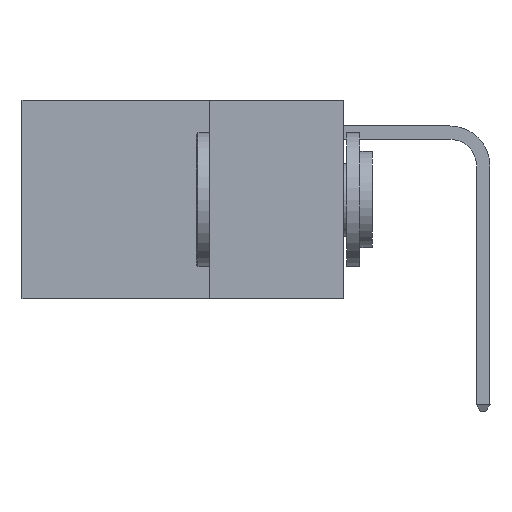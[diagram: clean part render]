
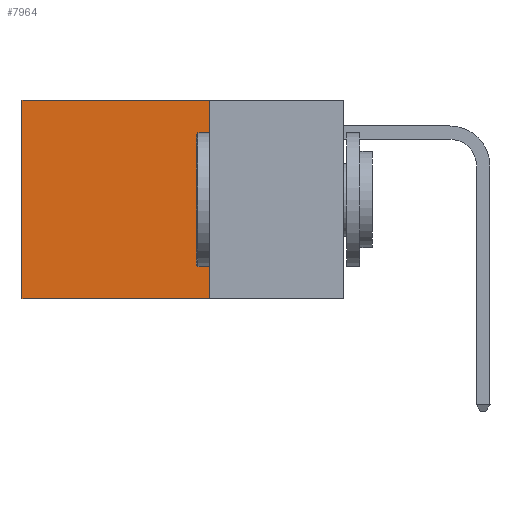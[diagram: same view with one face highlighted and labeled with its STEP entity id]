
A CAD part, left-side view. The second image highlights one B-rep face of the part: STEP entity #7964.
In plain terms, the highlighted planar face has unit normal (-1, 0, 0).
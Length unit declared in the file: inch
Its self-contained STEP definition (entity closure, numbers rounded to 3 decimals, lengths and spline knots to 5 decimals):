
#1226 = CARTESIAN_POINT ( 'NONE',  ( 0.2625, 0.25, 0. ) ) ;
#1303 = FACE_OUTER_BOUND ( 'NONE', #14444, .T. ) ;
#2228 = LINE ( 'NONE', #5620, #14779 ) ;
#3333 = DIRECTION ( 'NONE',  ( 0., 0., -1. ) ) ;
#3368 = EDGE_CURVE ( 'NONE', #9270, #14042, #2228, .T. ) ;
#3761 = EDGE_CURVE ( 'NONE', #9270, #8616, #7648, .T. ) ;
#3836 = DIRECTION ( 'NONE',  ( 0., 1., 0. ) ) ;
#4022 = CARTESIAN_POINT ( 'NONE',  ( 0.2625, 0.6, -0.37 ) ) ;
#4247 = VECTOR ( 'NONE', #3836, 39.37008 ) ;
#4575 = CARTESIAN_POINT ( 'NONE',  ( 0.2625, 0.6, 0. ) ) ;
#4822 = DIRECTION ( 'NONE',  ( 0., 0., -1. ) ) ;
#4838 = PLANE ( 'NONE',  #9672 ) ;
#5023 = CARTESIAN_POINT ( 'NONE',  ( 0.2625, 0.25, -0.37 ) ) ;
#5375 = VECTOR ( 'NONE', #4822, 39.37008 ) ;
#5493 = ORIENTED_EDGE ( 'NONE', *, *, #15145, .F. ) ;
#5620 = CARTESIAN_POINT ( 'NONE',  ( 0.2625, 0.25, 0. ) ) ;
#6087 = CARTESIAN_POINT ( 'NONE',  ( 0.2625, 0.6, 0. ) ) ;
#6207 = CARTESIAN_POINT ( 'NONE',  ( 0.2625, 0.25, 0. ) ) ;
#6238 = LINE ( 'NONE', #6087, #5375 ) ;
#7437 = DIRECTION ( 'NONE',  ( 1., 0., 0. ) ) ;
#7648 = LINE ( 'NONE', #10483, #7732 ) ;
#7732 = VECTOR ( 'NONE', #11745, 39.37008 ) ;
#7964 = ADVANCED_FACE ( 'NONE', ( #1303 ), #4838, .F. ) ;
#8307 = EDGE_CURVE ( 'NONE', #8616, #10285, #6238, .T. ) ;
#8616 = VERTEX_POINT ( 'NONE', #4575 ) ;
#9270 = VERTEX_POINT ( 'NONE', #6207 ) ;
#9672 = AXIS2_PLACEMENT_3D ( 'NONE', #1226, #7437, #11139 ) ;
#10285 = VERTEX_POINT ( 'NONE', #4022 ) ;
#10483 = CARTESIAN_POINT ( 'NONE',  ( 0.2625, 0.25, 0. ) ) ;
#11139 = DIRECTION ( 'NONE',  ( 0., 0., -1. ) ) ;
#11745 = DIRECTION ( 'NONE',  ( 0., 1., 0. ) ) ;
#13175 = ORIENTED_EDGE ( 'NONE', *, *, #3761, .T. ) ;
#13416 = CARTESIAN_POINT ( 'NONE',  ( 0.2625, 0.25, -0.37 ) ) ;
#14042 = VERTEX_POINT ( 'NONE', #13416 ) ;
#14444 = EDGE_LOOP ( 'NONE', ( #15398, #5493, #15547, #13175 ) ) ;
#14633 = LINE ( 'NONE', #5023, #4247 ) ;
#14779 = VECTOR ( 'NONE', #3333, 39.37008 ) ;
#15145 = EDGE_CURVE ( 'NONE', #14042, #10285, #14633, .T. ) ;
#15398 = ORIENTED_EDGE ( 'NONE', *, *, #8307, .T. ) ;
#15547 = ORIENTED_EDGE ( 'NONE', *, *, #3368, .F. ) ;
